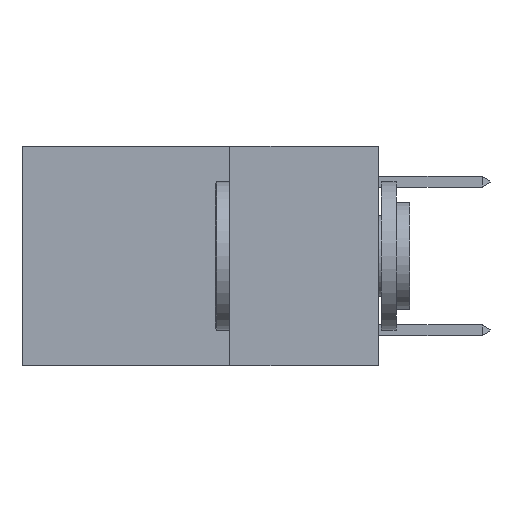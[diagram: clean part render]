
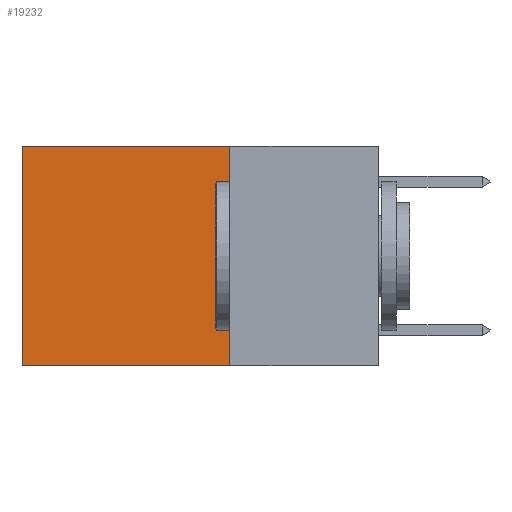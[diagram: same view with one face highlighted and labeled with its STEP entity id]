
A CAD part, left-side view. The second image highlights one B-rep face of the part: STEP entity #19232.
In plain terms, the highlighted planar face has unit normal (-1, 0, 0).
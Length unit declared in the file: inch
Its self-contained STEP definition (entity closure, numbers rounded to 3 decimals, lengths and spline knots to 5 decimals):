
#2386 = CARTESIAN_POINT ( 'NONE',  ( 0.2625, 0.25, 0. ) ) ;
#2914 = CARTESIAN_POINT ( 'NONE',  ( 0.2625, 0.25, -0.37 ) ) ;
#3102 = ORIENTED_EDGE ( 'NONE', *, *, #15953, .T. ) ;
#3587 = VECTOR ( 'NONE', #20560, 39.37008 ) ;
#4062 = DIRECTION ( 'NONE',  ( 0., 0., -1. ) ) ;
#4606 = ORIENTED_EDGE ( 'NONE', *, *, #19774, .F. ) ;
#4758 = VECTOR ( 'NONE', #15679, 39.37008 ) ;
#5203 = VECTOR ( 'NONE', #19427, 39.37008 ) ;
#5426 = EDGE_CURVE ( 'NONE', #7816, #15560, #18272, .T. ) ;
#7661 = LINE ( 'NONE', #15079, #5203 ) ;
#7816 = VERTEX_POINT ( 'NONE', #14703 ) ;
#8265 = LINE ( 'NONE', #12146, #4758 ) ;
#8400 = EDGE_LOOP ( 'NONE', ( #22276, #21207, #4606, #3102 ) ) ;
#8848 = VERTEX_POINT ( 'NONE', #2914 ) ;
#9046 = CARTESIAN_POINT ( 'NONE',  ( 0.2625, 0.6, 0. ) ) ;
#9624 = LINE ( 'NONE', #14985, #3587 ) ;
#12138 = AXIS2_PLACEMENT_3D ( 'NONE', #17398, #20683, #4062 ) ;
#12146 = CARTESIAN_POINT ( 'NONE',  ( 0.2625, 0.25, -0.37 ) ) ;
#12689 = EDGE_CURVE ( 'NONE', #8848, #15560, #8265, .T. ) ;
#14703 = CARTESIAN_POINT ( 'NONE',  ( 0.2625, 0.6, 0. ) ) ;
#14985 = CARTESIAN_POINT ( 'NONE',  ( 0.2625, 0.25, 0. ) ) ;
#15079 = CARTESIAN_POINT ( 'NONE',  ( 0.2625, 0.25, 0. ) ) ;
#15560 = VERTEX_POINT ( 'NONE', #19004 ) ;
#15679 = DIRECTION ( 'NONE',  ( 0., 1., 0. ) ) ;
#15953 = EDGE_CURVE ( 'NONE', #17392, #7816, #9624, .T. ) ;
#17164 = PLANE ( 'NONE',  #12138 ) ;
#17392 = VERTEX_POINT ( 'NONE', #2386 ) ;
#17398 = CARTESIAN_POINT ( 'NONE',  ( 0.2625, 0.25, 0. ) ) ;
#18272 = LINE ( 'NONE', #9046, #21886 ) ;
#18868 = FACE_OUTER_BOUND ( 'NONE', #8400, .T. ) ;
#19004 = CARTESIAN_POINT ( 'NONE',  ( 0.2625, 0.6, -0.37 ) ) ;
#19232 = ADVANCED_FACE ( 'NONE', ( #18868 ), #17164, .F. ) ;
#19427 = DIRECTION ( 'NONE',  ( 0., 0., -1. ) ) ;
#19774 = EDGE_CURVE ( 'NONE', #17392, #8848, #7661, .T. ) ;
#20560 = DIRECTION ( 'NONE',  ( 0., 1., 0. ) ) ;
#20683 = DIRECTION ( 'NONE',  ( 1., 0., 0. ) ) ;
#21207 = ORIENTED_EDGE ( 'NONE', *, *, #12689, .F. ) ;
#21886 = VECTOR ( 'NONE', #22060, 39.37008 ) ;
#22060 = DIRECTION ( 'NONE',  ( 0., 0., -1. ) ) ;
#22276 = ORIENTED_EDGE ( 'NONE', *, *, #5426, .T. ) ;
